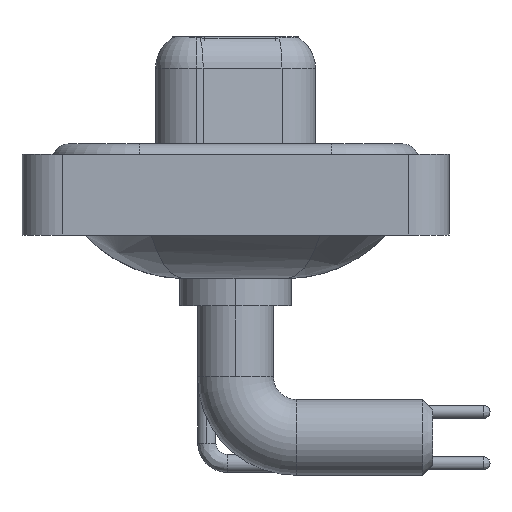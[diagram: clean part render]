
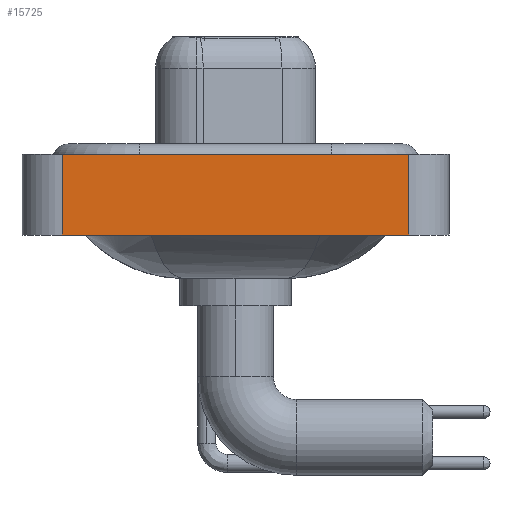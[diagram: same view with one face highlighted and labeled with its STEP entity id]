
A CAD part, left-side view. The second image highlights one B-rep face of the part: STEP entity #15725.
In plain terms, the highlighted planar face has unit normal (-1, 0, 0).
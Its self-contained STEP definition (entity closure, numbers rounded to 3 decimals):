
#309 = LINE ( 'NONE', #8110, #3231 ) ;
#1766 = VERTEX_POINT ( 'NONE', #3487 ) ;
#2643 = AXIS2_PLACEMENT_3D ( 'NONE', #19782, #16374, #13172 ) ;
#2872 = LINE ( 'NONE', #7760, #7775 ) ;
#3231 = VECTOR ( 'NONE', #14398, 1000. ) ;
#3487 = CARTESIAN_POINT ( 'NONE',  ( -7.3, -8.55, -3.6 ) ) ;
#3993 = VERTEX_POINT ( 'NONE', #7180 ) ;
#5141 = ORIENTED_EDGE ( 'NONE', *, *, #6054, .T. ) ;
#5229 = VECTOR ( 'NONE', #10461, 1000. ) ;
#5559 = CARTESIAN_POINT ( 'NONE',  ( -7.3, -8.55, 0.4 ) ) ;
#6054 = EDGE_CURVE ( 'NONE', #15792, #1766, #7258, .T. ) ;
#7180 = CARTESIAN_POINT ( 'NONE',  ( -7.3, -8.55, 0.4 ) ) ;
#7258 = LINE ( 'NONE', #19557, #5229 ) ;
#7760 = CARTESIAN_POINT ( 'NONE',  ( -7.3, -8.55, -3.6 ) ) ;
#7775 = VECTOR ( 'NONE', #9516, 1000. ) ;
#8110 = CARTESIAN_POINT ( 'NONE',  ( -7.3, 8.55, -3.6 ) ) ;
#8195 = VERTEX_POINT ( 'NONE', #9201 ) ;
#9201 = CARTESIAN_POINT ( 'NONE',  ( -7.3, 8.55, 0.4 ) ) ;
#9516 = DIRECTION ( 'NONE',  ( 0., 0., 1. ) ) ;
#9921 = ORIENTED_EDGE ( 'NONE', *, *, #18658, .T. ) ;
#10396 = CARTESIAN_POINT ( 'NONE',  ( -7.3, 8.55, -3.6 ) ) ;
#10461 = DIRECTION ( 'NONE',  ( 0., -1., 0. ) ) ;
#10877 = EDGE_CURVE ( 'NONE', #15792, #8195, #309, .T. ) ;
#12097 = EDGE_LOOP ( 'NONE', ( #9921, #15452, #12724, #5141 ) ) ;
#12724 = ORIENTED_EDGE ( 'NONE', *, *, #10877, .F. ) ;
#13172 = DIRECTION ( 'NONE',  ( 0., 0., 1. ) ) ;
#13280 = PLANE ( 'NONE',  #2643 ) ;
#14398 = DIRECTION ( 'NONE',  ( 0., 0., 1. ) ) ;
#14994 = DIRECTION ( 'NONE',  ( 0., -1., 0. ) ) ;
#15452 = ORIENTED_EDGE ( 'NONE', *, *, #16160, .F. ) ;
#15725 = ADVANCED_FACE ( 'NONE', ( #19481 ), #13280, .T. ) ;
#15792 = VERTEX_POINT ( 'NONE', #10396 ) ;
#16160 = EDGE_CURVE ( 'NONE', #8195, #3993, #18290, .T. ) ;
#16374 = DIRECTION ( 'NONE',  ( -1., 0., 0. ) ) ;
#18290 = LINE ( 'NONE', #5559, #19832 ) ;
#18658 = EDGE_CURVE ( 'NONE', #1766, #3993, #2872, .T. ) ;
#19481 = FACE_OUTER_BOUND ( 'NONE', #12097, .T. ) ;
#19557 = CARTESIAN_POINT ( 'NONE',  ( -7.3, -8.55, -3.6 ) ) ;
#19782 = CARTESIAN_POINT ( 'NONE',  ( -7.3, -8.55, -3.6 ) ) ;
#19832 = VECTOR ( 'NONE', #14994, 1000. ) ;
